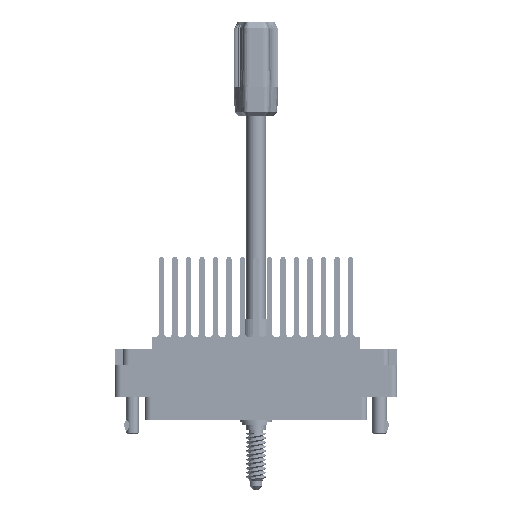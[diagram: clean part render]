
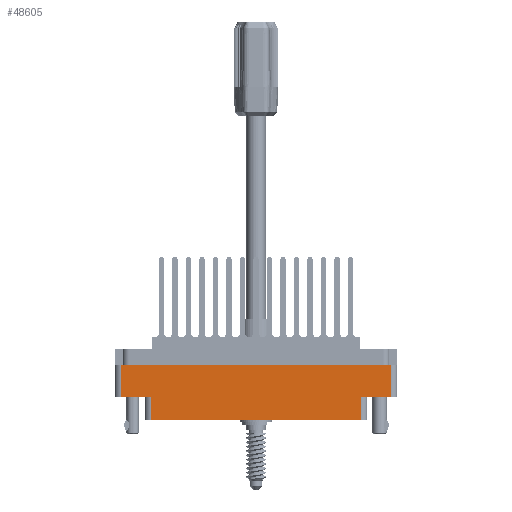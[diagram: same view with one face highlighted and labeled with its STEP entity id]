
A CAD part, front view. The second image highlights one B-rep face of the part: STEP entity #48605.
In plain terms, the highlighted planar face has unit normal (0, -1, 0).
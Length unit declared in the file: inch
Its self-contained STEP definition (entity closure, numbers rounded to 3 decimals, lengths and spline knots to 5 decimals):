
#509 = DIRECTION ( 'NONE',  ( 0., 0., 1. ) ) ;
#2112 = VERTEX_POINT ( 'NONE', #5604 ) ;
#2991 = EDGE_CURVE ( 'NONE', #48247, #85556, #15378, .T. ) ;
#3632 = DIRECTION ( 'NONE',  ( 0., 0., -1. ) ) ;
#5604 = CARTESIAN_POINT ( 'NONE',  ( 1.006, -0.617, -0.798 ) ) ;
#8562 = ORIENTED_EDGE ( 'NONE', *, *, #46661, .T. ) ;
#8752 = EDGE_LOOP ( 'NONE', ( #85635, #8562, #37056, #88939, #78316, #84007, #19035, #86932 ) ) ;
#10357 = VECTOR ( 'NONE', #36855, 39.37008 ) ;
#10918 = VERTEX_POINT ( 'NONE', #76350 ) ;
#13463 = CARTESIAN_POINT ( 'NONE',  ( 1.297, -0.617, -0.274 ) ) ;
#13558 = PLANE ( 'NONE',  #25072 ) ;
#15118 = VERTEX_POINT ( 'NONE', #62366 ) ;
#15378 = LINE ( 'NONE', #49900, #90723 ) ;
#16956 = CARTESIAN_POINT ( 'NONE',  ( -1.297, -0.617, -0.578 ) ) ;
#17604 = CARTESIAN_POINT ( 'NONE',  ( 0., -0.617, -0.578 ) ) ;
#18320 = EDGE_CURVE ( 'NONE', #10918, #2112, #70469, .T. ) ;
#19035 = ORIENTED_EDGE ( 'NONE', *, *, #2991, .F. ) ;
#20255 = CARTESIAN_POINT ( 'NONE',  ( -1.297, -0.617, -0.274 ) ) ;
#20911 = LINE ( 'NONE', #27204, #58577 ) ;
#24194 = DIRECTION ( 'NONE',  ( 0., 0., -1. ) ) ;
#24392 = LINE ( 'NONE', #87944, #35762 ) ;
#25072 = AXIS2_PLACEMENT_3D ( 'NONE', #42244, #50606, #93310 ) ;
#26306 = EDGE_CURVE ( 'NONE', #83140, #85556, #24392, .T. ) ;
#26451 = EDGE_CURVE ( 'NONE', #48247, #91587, #73559, .T. ) ;
#27204 = CARTESIAN_POINT ( 'NONE',  ( 1.006, -0.617, -0.578 ) ) ;
#29111 = VECTOR ( 'NONE', #24194, 39.37008 ) ;
#31095 = CARTESIAN_POINT ( 'NONE',  ( -1.006, -0.617, -0.578 ) ) ;
#31842 = CARTESIAN_POINT ( 'NONE',  ( -1.006, -0.617, -0.798 ) ) ;
#32009 = CARTESIAN_POINT ( 'NONE',  ( 1.297, -0.617, -0.578 ) ) ;
#34823 = EDGE_CURVE ( 'NONE', #2112, #15118, #20911, .T. ) ;
#35449 = LINE ( 'NONE', #88589, #10357 ) ;
#35762 = VECTOR ( 'NONE', #509, 39.37008 ) ;
#36855 = DIRECTION ( 'NONE',  ( 1., 0., 0. ) ) ;
#37056 = ORIENTED_EDGE ( 'NONE', *, *, #18320, .T. ) ;
#42244 = CARTESIAN_POINT ( 'NONE',  ( -1.359, -0.617, -0.798 ) ) ;
#46391 = VECTOR ( 'NONE', #55266, 39.37008 ) ;
#46661 = EDGE_CURVE ( 'NONE', #57478, #10918, #57715, .T. ) ;
#48247 = VERTEX_POINT ( 'NONE', #20255 ) ;
#48605 = ADVANCED_FACE ( 'NONE', ( #78210 ), #13558, .T. ) ;
#49900 = CARTESIAN_POINT ( 'NONE',  ( 0., -0.617, -0.274 ) ) ;
#50606 = DIRECTION ( 'NONE',  ( 0., -1., 0. ) ) ;
#55266 = DIRECTION ( 'NONE',  ( 1., 0., 0. ) ) ;
#57478 = VERTEX_POINT ( 'NONE', #31095 ) ;
#57715 = LINE ( 'NONE', #31842, #29111 ) ;
#58577 = VECTOR ( 'NONE', #71319, 39.37008 ) ;
#62366 = CARTESIAN_POINT ( 'NONE',  ( 1.006, -0.617, -0.578 ) ) ;
#62751 = VECTOR ( 'NONE', #76054, 39.37008 ) ;
#70469 = LINE ( 'NONE', #90294, #46391 ) ;
#71319 = DIRECTION ( 'NONE',  ( 0., 0., 1. ) ) ;
#71360 = EDGE_CURVE ( 'NONE', #91587, #57478, #35449, .T. ) ;
#72622 = EDGE_CURVE ( 'NONE', #83140, #15118, #77563, .T. ) ;
#73559 = LINE ( 'NONE', #76469, #83816 ) ;
#76054 = DIRECTION ( 'NONE',  ( -1., 0., 0. ) ) ;
#76350 = CARTESIAN_POINT ( 'NONE',  ( -1.006, -0.617, -0.798 ) ) ;
#76469 = CARTESIAN_POINT ( 'NONE',  ( -1.297, -0.617, -0.798 ) ) ;
#77563 = LINE ( 'NONE', #17604, #62751 ) ;
#78210 = FACE_OUTER_BOUND ( 'NONE', #8752, .T. ) ;
#78316 = ORIENTED_EDGE ( 'NONE', *, *, #72622, .F. ) ;
#83140 = VERTEX_POINT ( 'NONE', #32009 ) ;
#83816 = VECTOR ( 'NONE', #3632, 39.37008 ) ;
#84007 = ORIENTED_EDGE ( 'NONE', *, *, #26306, .T. ) ;
#85556 = VERTEX_POINT ( 'NONE', #13463 ) ;
#85635 = ORIENTED_EDGE ( 'NONE', *, *, #71360, .T. ) ;
#86932 = ORIENTED_EDGE ( 'NONE', *, *, #26451, .T. ) ;
#87772 = DIRECTION ( 'NONE',  ( 1., 0., 0. ) ) ;
#87944 = CARTESIAN_POINT ( 'NONE',  ( 1.297, -0.617, -0.798 ) ) ;
#88589 = CARTESIAN_POINT ( 'NONE',  ( 0., -0.617, -0.578 ) ) ;
#88939 = ORIENTED_EDGE ( 'NONE', *, *, #34823, .T. ) ;
#90294 = CARTESIAN_POINT ( 'NONE',  ( -1.359, -0.617, -0.798 ) ) ;
#90723 = VECTOR ( 'NONE', #87772, 39.37008 ) ;
#91587 = VERTEX_POINT ( 'NONE', #16956 ) ;
#93310 = DIRECTION ( 'NONE',  ( 0., 0., -1. ) ) ;
